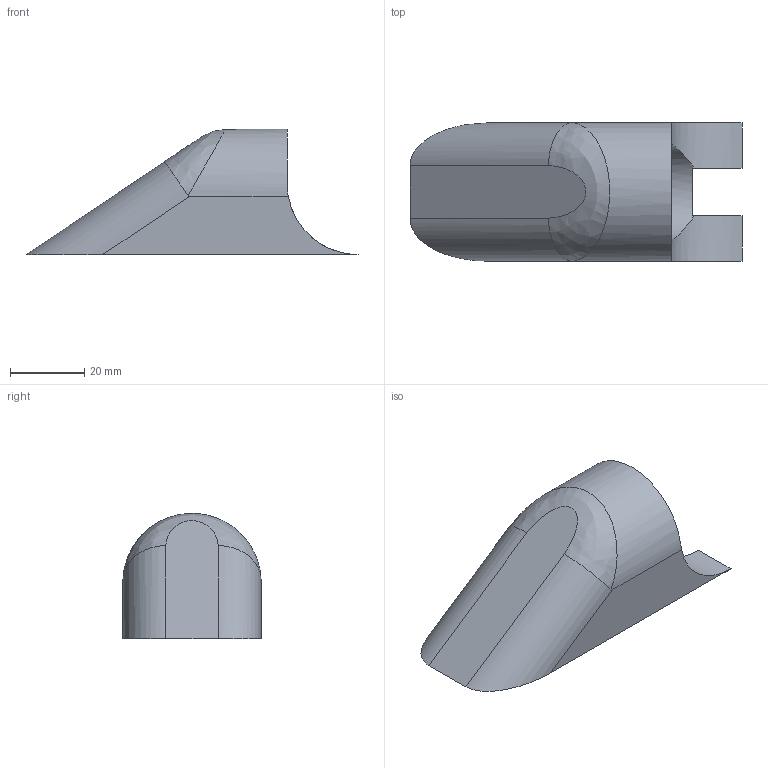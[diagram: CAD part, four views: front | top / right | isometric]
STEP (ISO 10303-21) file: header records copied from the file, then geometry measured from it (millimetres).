
FILE_DESCRIPTION (( 'STEP AP214' ), '1' );
FILE_NAME ('Unbuffered_Pistol_1.STEP', '2013-09-01T16:58:04', ( 'Asher' ), ( '' ), 'SwSTEP 2.0', 'SolidWorks 2013', '' );
FILE_SCHEMA (( 'AUTOMOTIVE_DESIGN' ));
Length unit declared in the file: millimetre
Products named in the file (1): Unbuffered_Pistol_1
Bounding box: 89.22 x 37.13 x 33.66 mm (x, y, z)
Volume: 51824.7 mm3; surface area: 9878.3 mm2
Topology: 1 solids, 1 shells, 24 faces, 84 edges, 62 vertices
Faces by surface type: sphere 9, plane 8, cylinder 6, bspline 1
Entity records: 955 total; most frequent: CARTESIAN_POINT 349, DIRECTION 118, ORIENTED_EDGE 114, EDGE_CURVE 57, AXIS2_PLACEMENT_3D 49, VERTEX_POINT 44, EDGE_LOOP 33, CIRCLE 25
